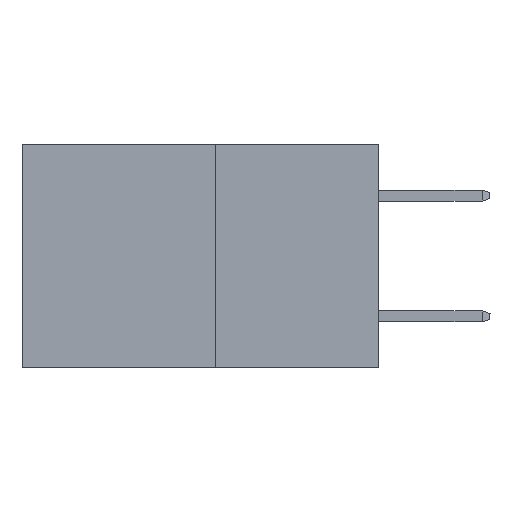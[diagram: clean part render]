
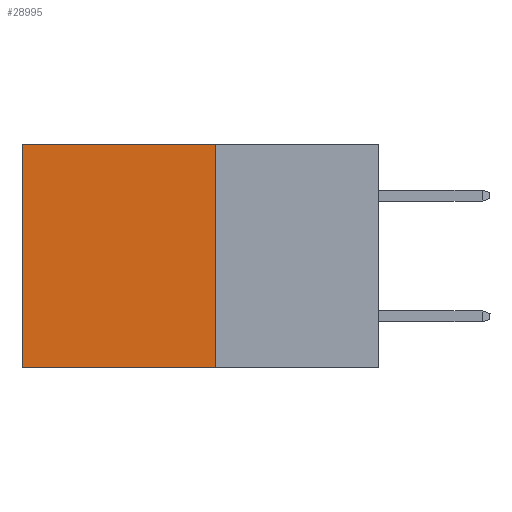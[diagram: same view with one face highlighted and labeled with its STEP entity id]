
A CAD part, left-side view. The second image highlights one B-rep face of the part: STEP entity #28995.
In plain terms, the highlighted planar face has unit normal (-1, 0, 0).
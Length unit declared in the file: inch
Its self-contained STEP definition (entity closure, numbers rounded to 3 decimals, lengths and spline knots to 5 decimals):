
#548 = VERTEX_POINT ( 'NONE', #19879 ) ;
#634 = CARTESIAN_POINT ( 'NONE',  ( 0.277, 0.27, -0.37 ) ) ;
#763 = DIRECTION ( 'NONE',  ( 0., 0., -1. ) ) ;
#1492 = DIRECTION ( 'NONE',  ( 0., 1., 0. ) ) ;
#2255 = LINE ( 'NONE', #18328, #19281 ) ;
#2693 = EDGE_LOOP ( 'NONE', ( #27669, #26464, #11539, #10283 ) ) ;
#5505 = PLANE ( 'NONE',  #20421 ) ;
#5573 = FACE_OUTER_BOUND ( 'NONE', #2693, .T. ) ;
#5877 = VECTOR ( 'NONE', #1492, 39.37008 ) ;
#7705 = VERTEX_POINT ( 'NONE', #20220 ) ;
#9100 = LINE ( 'NONE', #14842, #26632 ) ;
#9944 = EDGE_CURVE ( 'NONE', #27497, #548, #2255, .T. ) ;
#10173 = CARTESIAN_POINT ( 'NONE',  ( 0.277, 0.27, -0.37 ) ) ;
#10283 = ORIENTED_EDGE ( 'NONE', *, *, #18603, .T. ) ;
#11539 = ORIENTED_EDGE ( 'NONE', *, *, #28267, .F. ) ;
#12506 = DIRECTION ( 'NONE',  ( 0., 0., -1. ) ) ;
#13080 = CARTESIAN_POINT ( 'NONE',  ( 0.277, 0.27, -0.37 ) ) ;
#14346 = VECTOR ( 'NONE', #763, 39.37008 ) ;
#14842 = CARTESIAN_POINT ( 'NONE',  ( 0.277, 0.27, 0. ) ) ;
#15976 = DIRECTION ( 'NONE',  ( 0., 0., -1. ) ) ;
#18328 = CARTESIAN_POINT ( 'NONE',  ( 0.277, 0.59, -0.37 ) ) ;
#18506 = VERTEX_POINT ( 'NONE', #634 ) ;
#18603 = EDGE_CURVE ( 'NONE', #7705, #27497, #9100, .T. ) ;
#19055 = CARTESIAN_POINT ( 'NONE',  ( 0.277, 0.59, 0. ) ) ;
#19281 = VECTOR ( 'NONE', #15976, 39.37008 ) ;
#19879 = CARTESIAN_POINT ( 'NONE',  ( 0.277, 0.59, -0.37 ) ) ;
#20220 = CARTESIAN_POINT ( 'NONE',  ( 0.277, 0.27, 0. ) ) ;
#20421 = AXIS2_PLACEMENT_3D ( 'NONE', #10173, #26189, #12506 ) ;
#20491 = LINE ( 'NONE', #23783, #14346 ) ;
#23438 = EDGE_CURVE ( 'NONE', #18506, #548, #23564, .T. ) ;
#23564 = LINE ( 'NONE', #13080, #5877 ) ;
#23783 = CARTESIAN_POINT ( 'NONE',  ( 0.277, 0.27, -0.37 ) ) ;
#26189 = DIRECTION ( 'NONE',  ( 1., 0., 0. ) ) ;
#26464 = ORIENTED_EDGE ( 'NONE', *, *, #23438, .F. ) ;
#26632 = VECTOR ( 'NONE', #28473, 39.37008 ) ;
#27497 = VERTEX_POINT ( 'NONE', #19055 ) ;
#27669 = ORIENTED_EDGE ( 'NONE', *, *, #9944, .T. ) ;
#28267 = EDGE_CURVE ( 'NONE', #7705, #18506, #20491, .T. ) ;
#28473 = DIRECTION ( 'NONE',  ( 0., 1., 0. ) ) ;
#28995 = ADVANCED_FACE ( 'NONE', ( #5573 ), #5505, .F. ) ;
